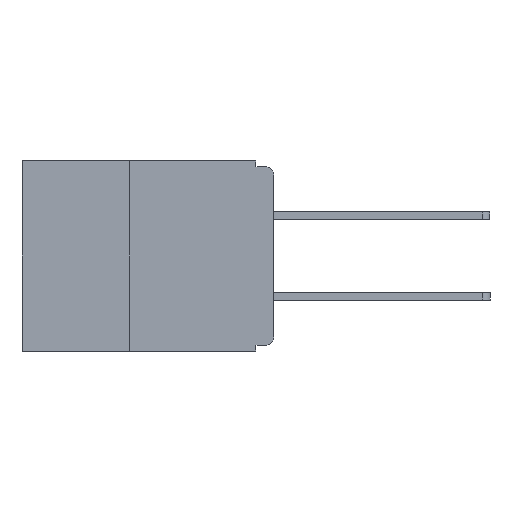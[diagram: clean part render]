
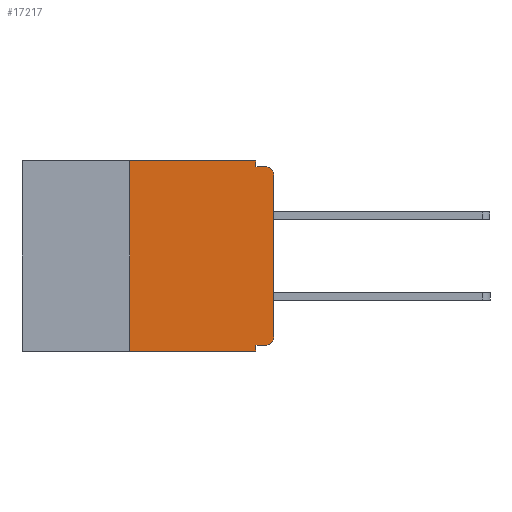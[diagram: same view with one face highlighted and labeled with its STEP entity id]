
A CAD part, left-side view. The second image highlights one B-rep face of the part: STEP entity #17217.
In plain terms, the highlighted planar face has unit normal (-1, 0, 0).
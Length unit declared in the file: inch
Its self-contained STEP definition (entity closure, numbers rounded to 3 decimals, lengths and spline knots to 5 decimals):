
#217 = LINE ( 'NONE', #28465, #28880 ) ;
#307 = VERTEX_POINT ( 'NONE', #19064 ) ;
#467 = ORIENTED_EDGE ( 'NONE', *, *, #8285, .F. ) ;
#473 = ORIENTED_EDGE ( 'NONE', *, *, #5120, .F. ) ;
#1442 = DIRECTION ( 'NONE',  ( 0., 0., 1. ) ) ;
#1872 = VECTOR ( 'NONE', #12890, 39.37008 ) ;
#2354 = PLANE ( 'NONE',  #22080 ) ;
#3178 = VERTEX_POINT ( 'NONE', #21807 ) ;
#3250 = VERTEX_POINT ( 'NONE', #17368 ) ;
#4758 = CARTESIAN_POINT ( 'NONE',  ( 0., 0.437, 0. ) ) ;
#5053 = CIRCLE ( 'NONE', #22843, 0.015 ) ;
#5067 = FACE_OUTER_BOUND ( 'NONE', #28147, .T. ) ;
#5120 = EDGE_CURVE ( 'NONE', #307, #3178, #19435, .T. ) ;
#5210 = EDGE_CURVE ( 'NONE', #6071, #10481, #23198, .T. ) ;
#5561 = CARTESIAN_POINT ( 'NONE',  ( 0., 0.015, -0.01 ) ) ;
#5650 = DIRECTION ( 'NONE',  ( 0., 0., 1. ) ) ;
#6071 = VERTEX_POINT ( 'NONE', #16966 ) ;
#6241 = VERTEX_POINT ( 'NONE', #5561 ) ;
#6436 = ORIENTED_EDGE ( 'NONE', *, *, #7483, .F. ) ;
#6726 = VECTOR ( 'NONE', #24935, 39.37008 ) ;
#7156 = DIRECTION ( 'NONE',  ( 1., 0., 0. ) ) ;
#7297 = VERTEX_POINT ( 'NONE', #25733 ) ;
#7483 = EDGE_CURVE ( 'NONE', #19400, #307, #217, .T. ) ;
#7514 = ORIENTED_EDGE ( 'NONE', *, *, #7973, .T. ) ;
#7712 = ORIENTED_EDGE ( 'NONE', *, *, #23951, .T. ) ;
#7764 = CARTESIAN_POINT ( 'NONE',  ( 0., 0.031, -0.01 ) ) ;
#7973 = EDGE_CURVE ( 'NONE', #3250, #6241, #5053, .T. ) ;
#8285 = EDGE_CURVE ( 'NONE', #10481, #7297, #9133, .T. ) ;
#8649 = EDGE_CURVE ( 'NONE', #24579, #3250, #28158, .T. ) ;
#8720 = ORIENTED_EDGE ( 'NONE', *, *, #27516, .T. ) ;
#9133 = LINE ( 'NONE', #22135, #14440 ) ;
#9410 = AXIS2_PLACEMENT_3D ( 'NONE', #11997, #27391, #14227 ) ;
#9800 = DIRECTION ( 'NONE',  ( 0., 1., 0. ) ) ;
#9989 = CARTESIAN_POINT ( 'NONE',  ( 0., 0., -0.32 ) ) ;
#10481 = VERTEX_POINT ( 'NONE', #18589 ) ;
#11713 = CARTESIAN_POINT ( 'NONE',  ( 0., 0.437, -0.33 ) ) ;
#11785 = EDGE_CURVE ( 'NONE', #17381, #6241, #25666, .T. ) ;
#11997 = CARTESIAN_POINT ( 'NONE',  ( 0., 0.015, -0.305 ) ) ;
#12487 = CARTESIAN_POINT ( 'NONE',  ( 0., 0.015, -0.025 ) ) ;
#12804 = CARTESIAN_POINT ( 'NONE',  ( 0., 0.437, 0. ) ) ;
#12890 = DIRECTION ( 'NONE',  ( 0., -1., 0. ) ) ;
#14013 = CARTESIAN_POINT ( 'NONE',  ( 0., 0., -0.305 ) ) ;
#14227 = DIRECTION ( 'NONE',  ( 0., 0., -1. ) ) ;
#14440 = VECTOR ( 'NONE', #22323, 39.37008 ) ;
#14703 = DIRECTION ( 'NONE',  ( 0., 0., -1. ) ) ;
#15734 = CIRCLE ( 'NONE', #9410, 0.015 ) ;
#15918 = CARTESIAN_POINT ( 'NONE',  ( 0., 0.031, 0. ) ) ;
#16452 = DIRECTION ( 'NONE',  ( 0., -1., 0. ) ) ;
#16966 = CARTESIAN_POINT ( 'NONE',  ( 0., 0.015, -0.32 ) ) ;
#17217 = ADVANCED_FACE ( 'NONE', ( #5067 ), #2354, .F. ) ;
#17320 = VECTOR ( 'NONE', #9800, 39.37008 ) ;
#17368 = CARTESIAN_POINT ( 'NONE',  ( 0., 0., -0.025 ) ) ;
#17381 = VERTEX_POINT ( 'NONE', #7764 ) ;
#18175 = DIRECTION ( 'NONE',  ( 0., 0., -1. ) ) ;
#18589 = CARTESIAN_POINT ( 'NONE',  ( 0., 0.031, -0.32 ) ) ;
#18753 = LINE ( 'NONE', #11713, #6726 ) ;
#19064 = CARTESIAN_POINT ( 'NONE',  ( 0., 0.25, 0. ) ) ;
#19400 = VERTEX_POINT ( 'NONE', #27572 ) ;
#19435 = LINE ( 'NONE', #12804, #1872 ) ;
#21455 = CARTESIAN_POINT ( 'NONE',  ( 0., 0., 0. ) ) ;
#21681 = VECTOR ( 'NONE', #5650, 39.37008 ) ;
#21807 = CARTESIAN_POINT ( 'NONE',  ( 0., 0.031, 0. ) ) ;
#21812 = LINE ( 'NONE', #15918, #28298 ) ;
#22080 = AXIS2_PLACEMENT_3D ( 'NONE', #4758, #7156, #22825 ) ;
#22135 = CARTESIAN_POINT ( 'NONE',  ( 0., 0.031, -0.33 ) ) ;
#22323 = DIRECTION ( 'NONE',  ( 0., 0., -1. ) ) ;
#22825 = DIRECTION ( 'NONE',  ( 0., 0., -1. ) ) ;
#22843 = AXIS2_PLACEMENT_3D ( 'NONE', #12487, #27871, #14703 ) ;
#23025 = CARTESIAN_POINT ( 'NONE',  ( 0., 0., -0.01 ) ) ;
#23138 = ORIENTED_EDGE ( 'NONE', *, *, #5210, .F. ) ;
#23198 = LINE ( 'NONE', #9989, #17320 ) ;
#23951 = EDGE_CURVE ( 'NONE', #19400, #7297, #18753, .T. ) ;
#24511 = EDGE_CURVE ( 'NONE', #3178, #17381, #21812, .T. ) ;
#24579 = VERTEX_POINT ( 'NONE', #14013 ) ;
#24935 = DIRECTION ( 'NONE',  ( 0., -1., 0. ) ) ;
#24990 = VECTOR ( 'NONE', #16452, 39.37008 ) ;
#25666 = LINE ( 'NONE', #23025, #24990 ) ;
#25733 = CARTESIAN_POINT ( 'NONE',  ( 0., 0.031, -0.33 ) ) ;
#26361 = ORIENTED_EDGE ( 'NONE', *, *, #11785, .F. ) ;
#27391 = DIRECTION ( 'NONE',  ( -1., 0., 0. ) ) ;
#27516 = EDGE_CURVE ( 'NONE', #6071, #24579, #15734, .T. ) ;
#27567 = ORIENTED_EDGE ( 'NONE', *, *, #24511, .F. ) ;
#27572 = CARTESIAN_POINT ( 'NONE',  ( 0., 0.25, -0.33 ) ) ;
#27871 = DIRECTION ( 'NONE',  ( -1., 0., 0. ) ) ;
#28147 = EDGE_LOOP ( 'NONE', ( #28707, #7514, #26361, #27567, #473, #6436, #7712, #467, #23138, #8720 ) ) ;
#28158 = LINE ( 'NONE', #21455, #21681 ) ;
#28298 = VECTOR ( 'NONE', #18175, 39.37008 ) ;
#28465 = CARTESIAN_POINT ( 'NONE',  ( 0., 0.25, -0.33 ) ) ;
#28707 = ORIENTED_EDGE ( 'NONE', *, *, #8649, .T. ) ;
#28880 = VECTOR ( 'NONE', #1442, 39.37008 ) ;
